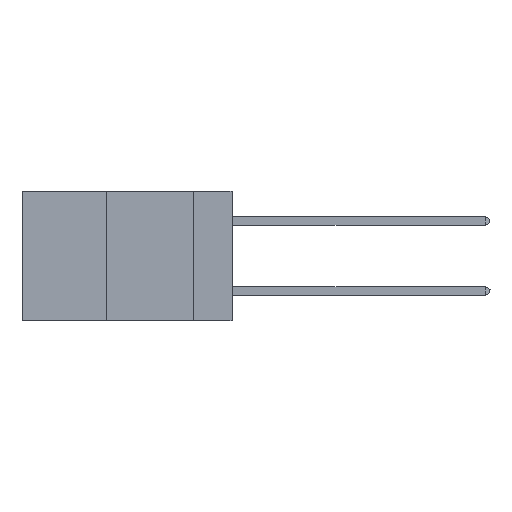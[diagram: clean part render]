
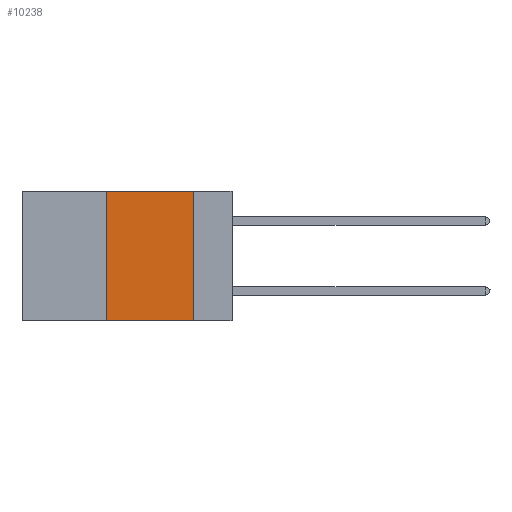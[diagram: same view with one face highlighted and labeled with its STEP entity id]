
A CAD part, left-side view. The second image highlights one B-rep face of the part: STEP entity #10238.
In plain terms, the highlighted planar face has unit normal (-1, 0, 0).
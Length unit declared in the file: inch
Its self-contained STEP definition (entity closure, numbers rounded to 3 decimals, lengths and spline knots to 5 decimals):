
#1423 = DIRECTION ( 'NONE',  ( 0., 0., -1. ) ) ;
#2618 = EDGE_LOOP ( 'NONE', ( #7229, #23285, #18311, #8098 ) ) ;
#2668 = CARTESIAN_POINT ( 'NONE',  ( 0., 0.6, -0.37 ) ) ;
#3100 = EDGE_CURVE ( 'NONE', #14730, #4189, #22914, .T. ) ;
#3630 = VERTEX_POINT ( 'NONE', #15766 ) ;
#4117 = DIRECTION ( 'NONE',  ( 0., 0., -1. ) ) ;
#4189 = VERTEX_POINT ( 'NONE', #12096 ) ;
#5643 = EDGE_CURVE ( 'NONE', #20231, #3630, #12484, .T. ) ;
#6394 = DIRECTION ( 'NONE',  ( 0., -1., 0. ) ) ;
#6553 = LINE ( 'NONE', #21066, #12198 ) ;
#6837 = CARTESIAN_POINT ( 'NONE',  ( 0., 0.6, 0. ) ) ;
#7229 = ORIENTED_EDGE ( 'NONE', *, *, #13070, .F. ) ;
#7437 = VECTOR ( 'NONE', #6394, 39.37008 ) ;
#8098 = ORIENTED_EDGE ( 'NONE', *, *, #5643, .T. ) ;
#8359 = DIRECTION ( 'NONE',  ( 0., 0., 1. ) ) ;
#8550 = DIRECTION ( 'NONE',  ( 1., 0., 0. ) ) ;
#8689 = DIRECTION ( 'NONE',  ( 0., -1., 0. ) ) ;
#9811 = AXIS2_PLACEMENT_3D ( 'NONE', #21853, #8550, #1423 ) ;
#10083 = CARTESIAN_POINT ( 'NONE',  ( 0., 0.36, 0. ) ) ;
#10238 = ADVANCED_FACE ( 'NONE', ( #15588 ), #19829, .F. ) ;
#12096 = CARTESIAN_POINT ( 'NONE',  ( 0., 0.11, 0. ) ) ;
#12107 = VECTOR ( 'NONE', #8359, 39.37008 ) ;
#12198 = VECTOR ( 'NONE', #4117, 39.37008 ) ;
#12484 = LINE ( 'NONE', #2668, #7437 ) ;
#13070 = EDGE_CURVE ( 'NONE', #4189, #3630, #6553, .T. ) ;
#13442 = CARTESIAN_POINT ( 'NONE',  ( 0., 0.36, -0.37 ) ) ;
#14730 = VERTEX_POINT ( 'NONE', #23220 ) ;
#15588 = FACE_OUTER_BOUND ( 'NONE', #2618, .T. ) ;
#15766 = CARTESIAN_POINT ( 'NONE',  ( 0., 0.11, -0.37 ) ) ;
#15965 = LINE ( 'NONE', #10083, #12107 ) ;
#17890 = VECTOR ( 'NONE', #8689, 39.37008 ) ;
#17892 = EDGE_CURVE ( 'NONE', #20231, #14730, #15965, .T. ) ;
#18311 = ORIENTED_EDGE ( 'NONE', *, *, #17892, .F. ) ;
#19829 = PLANE ( 'NONE',  #9811 ) ;
#20231 = VERTEX_POINT ( 'NONE', #13442 ) ;
#21066 = CARTESIAN_POINT ( 'NONE',  ( 0., 0.11, 0. ) ) ;
#21853 = CARTESIAN_POINT ( 'NONE',  ( 0., 0.6, 0. ) ) ;
#22914 = LINE ( 'NONE', #6837, #17890 ) ;
#23220 = CARTESIAN_POINT ( 'NONE',  ( 0., 0.36, 0. ) ) ;
#23285 = ORIENTED_EDGE ( 'NONE', *, *, #3100, .F. ) ;
